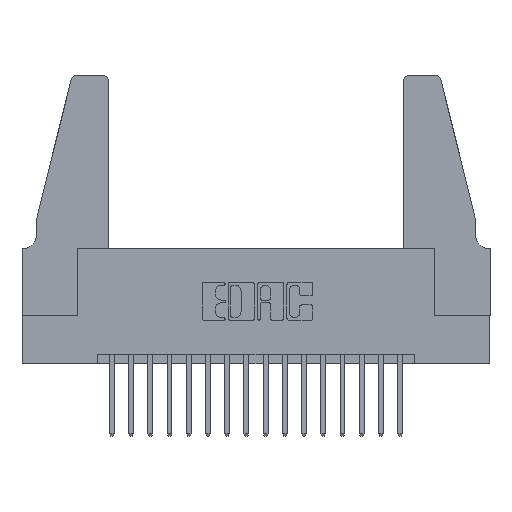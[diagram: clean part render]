
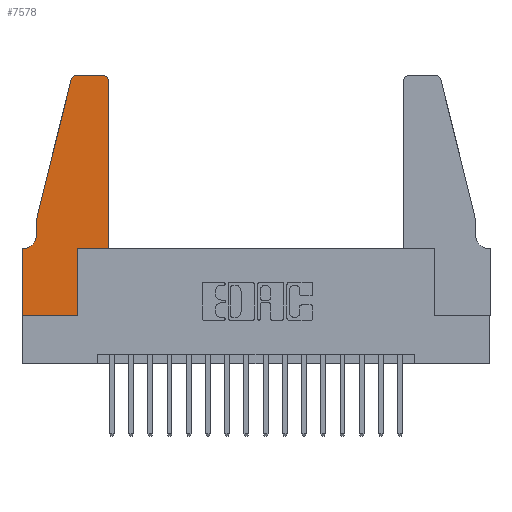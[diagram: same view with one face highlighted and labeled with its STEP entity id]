
A CAD part, top view. The second image highlights one B-rep face of the part: STEP entity #7578.
In plain terms, the highlighted planar face has unit normal (0, 0, 1).
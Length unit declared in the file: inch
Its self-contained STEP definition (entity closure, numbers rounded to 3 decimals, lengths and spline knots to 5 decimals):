
#6 = CARTESIAN_POINT ( 'NONE',  ( 0.0755, 0.5, 0.37 ) ) ;
#129 = CARTESIAN_POINT ( 'NONE',  ( 0.4205, 1.22, 0.37 ) ) ;
#446 = ORIENTED_EDGE ( 'NONE', *, *, #8183, .T. ) ;
#811 = CARTESIAN_POINT ( 'NONE',  ( 0., 0.35, 0.37 ) ) ;
#850 = CARTESIAN_POINT ( 'NONE',  ( 0.4205, 1.25, 0.37 ) ) ;
#881 = VECTOR ( 'NONE', #11920, 39.37008 ) ;
#1114 = CARTESIAN_POINT ( 'NONE',  ( 0.284, 1.22, 0.37 ) ) ;
#1154 = ORIENTED_EDGE ( 'NONE', *, *, #18149, .T. ) ;
#1182 = CARTESIAN_POINT ( 'NONE',  ( 0.4505, 0.35, 0.37 ) ) ;
#1520 = DIRECTION ( 'NONE',  ( 1., 0., 0. ) ) ;
#1636 = EDGE_CURVE ( 'NONE', #12787, #14306, #3996, .T. ) ;
#1684 = LINE ( 'NONE', #9466, #16262 ) ;
#1925 = EDGE_CURVE ( 'NONE', #4244, #3979, #17481, .T. ) ;
#2130 = CARTESIAN_POINT ( 'NONE',  ( 0., 0.35, 0.37 ) ) ;
#2363 = VECTOR ( 'NONE', #8413, 39.37008 ) ;
#2592 = CARTESIAN_POINT ( 'NONE',  ( 0.0055, 0.35, 0.37 ) ) ;
#2676 = CARTESIAN_POINT ( 'NONE',  ( 0.2865, 0.35, 0.37 ) ) ;
#2794 = CARTESIAN_POINT ( 'NONE',  ( 0.284, 1.25, 0.37 ) ) ;
#2969 = AXIS2_PLACEMENT_3D ( 'NONE', #1114, #8069, #10960 ) ;
#3422 = ORIENTED_EDGE ( 'NONE', *, *, #1636, .T. ) ;
#3979 = VERTEX_POINT ( 'NONE', #11394 ) ;
#3996 = LINE ( 'NONE', #12353, #13262 ) ;
#4066 = DIRECTION ( 'NONE',  ( 0., 1., 0. ) ) ;
#4141 = ORIENTED_EDGE ( 'NONE', *, *, #5455, .T. ) ;
#4175 = CARTESIAN_POINT ( 'NONE',  ( 0.25487, 1.22718, 0.37 ) ) ;
#4244 = VERTEX_POINT ( 'NONE', #1182 ) ;
#4346 = EDGE_CURVE ( 'NONE', #7268, #17238, #17404, .T. ) ;
#4402 = CARTESIAN_POINT ( 'NONE',  ( 0.0755, 0.42, 0.37 ) ) ;
#4586 = LINE ( 'NONE', #17491, #881 ) ;
#4915 = PLANE ( 'NONE',  #17980 ) ;
#5394 = VECTOR ( 'NONE', #4066, 39.37008 ) ;
#5455 = EDGE_CURVE ( 'NONE', #15726, #9981, #13923, .T. ) ;
#5701 = CARTESIAN_POINT ( 'NONE',  ( 0.0055, 0.42, 0.37 ) ) ;
#5777 = LINE ( 'NONE', #5840, #15089 ) ;
#5840 = CARTESIAN_POINT ( 'NONE',  ( 0.0755, 0.5, 0.37 ) ) ;
#5896 = CARTESIAN_POINT ( 'NONE',  ( 0., 0., 0.37 ) ) ;
#6059 = ORIENTED_EDGE ( 'NONE', *, *, #4346, .T. ) ;
#6671 = ORIENTED_EDGE ( 'NONE', *, *, #8958, .T. ) ;
#6711 = CARTESIAN_POINT ( 'NONE',  ( 0.4505, 0.35, 0.37 ) ) ;
#6892 = EDGE_CURVE ( 'NONE', #8736, #8867, #4586, .T. ) ;
#7268 = VERTEX_POINT ( 'NONE', #2592 ) ;
#7578 = ADVANCED_FACE ( 'NONE', ( #15820 ), #4915, .T. ) ;
#8048 = CARTESIAN_POINT ( 'NONE',  ( 0.2865, 0.35, 0.37 ) ) ;
#8069 = DIRECTION ( 'NONE',  ( 0., 0., 1. ) ) ;
#8148 = VECTOR ( 'NONE', #16765, 39.37008 ) ;
#8183 = EDGE_CURVE ( 'NONE', #8867, #10814, #10039, .T. ) ;
#8195 = EDGE_CURVE ( 'NONE', #17238, #12787, #1684, .T. ) ;
#8413 = DIRECTION ( 'NONE',  ( 1., 0., 0. ) ) ;
#8728 = VERTEX_POINT ( 'NONE', #8048 ) ;
#8736 = VERTEX_POINT ( 'NONE', #850 ) ;
#8867 = VERTEX_POINT ( 'NONE', #2794 ) ;
#8958 = EDGE_CURVE ( 'NONE', #14306, #8728, #9372, .T. ) ;
#9372 = LINE ( 'NONE', #2676, #5394 ) ;
#9466 = CARTESIAN_POINT ( 'NONE',  ( 0., 0., 0.37 ) ) ;
#9530 = DIRECTION ( 'NONE',  ( 0., -1., 0. ) ) ;
#9537 = EDGE_CURVE ( 'NONE', #9981, #7268, #10000, .T. ) ;
#9835 = LINE ( 'NONE', #12566, #2363 ) ;
#9981 = VERTEX_POINT ( 'NONE', #4402 ) ;
#10000 = CIRCLE ( 'NONE', #14908, 0.07 ) ;
#10039 = CIRCLE ( 'NONE', #2969, 0.03 ) ;
#10134 = ORIENTED_EDGE ( 'NONE', *, *, #1925, .T. ) ;
#10814 = VERTEX_POINT ( 'NONE', #4175 ) ;
#10960 = DIRECTION ( 'NONE',  ( 1., 0., 0. ) ) ;
#11394 = CARTESIAN_POINT ( 'NONE',  ( 0.4505, 1.22, 0.37 ) ) ;
#11684 = DIRECTION ( 'NONE',  ( -1., 0., 0. ) ) ;
#11920 = DIRECTION ( 'NONE',  ( -1., 0., 0. ) ) ;
#11992 = AXIS2_PLACEMENT_3D ( 'NONE', #129, #12857, #1520 ) ;
#12176 = VECTOR ( 'NONE', #12355, 39.37008 ) ;
#12353 = CARTESIAN_POINT ( 'NONE',  ( 0., 0., 0.37 ) ) ;
#12355 = DIRECTION ( 'NONE',  ( 0., 1., 0. ) ) ;
#12366 = EDGE_LOOP ( 'NONE', ( #12546, #446, #1154, #4141, #17890, #6059, #16382, #3422, #6671, #12944, #10134, #13856 ) ) ;
#12546 = ORIENTED_EDGE ( 'NONE', *, *, #6892, .T. ) ;
#12566 = CARTESIAN_POINT ( 'NONE',  ( 0.4505, 0.35, 0.37 ) ) ;
#12585 = CARTESIAN_POINT ( 'NONE',  ( 0.0755, 0.5, 0.37 ) ) ;
#12787 = VERTEX_POINT ( 'NONE', #5896 ) ;
#12857 = DIRECTION ( 'NONE',  ( 0., 0., 1. ) ) ;
#12944 = ORIENTED_EDGE ( 'NONE', *, *, #17320, .T. ) ;
#13155 = EDGE_CURVE ( 'NONE', #3979, #8736, #16408, .T. ) ;
#13262 = VECTOR ( 'NONE', #16579, 39.37008 ) ;
#13385 = CARTESIAN_POINT ( 'NONE',  ( 0.2865, 0., 0.37 ) ) ;
#13482 = DIRECTION ( 'NONE',  ( 1., 0., 0. ) ) ;
#13666 = CARTESIAN_POINT ( 'NONE',  ( 0.0755, 0.35, 0.37 ) ) ;
#13856 = ORIENTED_EDGE ( 'NONE', *, *, #13155, .T. ) ;
#13923 = LINE ( 'NONE', #6, #8148 ) ;
#14306 = VERTEX_POINT ( 'NONE', #13385 ) ;
#14908 = AXIS2_PLACEMENT_3D ( 'NONE', #5701, #15600, #11684 ) ;
#14922 = DIRECTION ( 'NONE',  ( 0., 0., 1. ) ) ;
#14960 = VECTOR ( 'NONE', #17962, 39.37008 ) ;
#15089 = VECTOR ( 'NONE', #17344, 39.37008 ) ;
#15600 = DIRECTION ( 'NONE',  ( 0., 0., -1. ) ) ;
#15726 = VERTEX_POINT ( 'NONE', #12585 ) ;
#15820 = FACE_OUTER_BOUND ( 'NONE', #12366, .T. ) ;
#16262 = VECTOR ( 'NONE', #9530, 39.37008 ) ;
#16382 = ORIENTED_EDGE ( 'NONE', *, *, #8195, .T. ) ;
#16408 = CIRCLE ( 'NONE', #11992, 0.03 ) ;
#16579 = DIRECTION ( 'NONE',  ( 1., 0., 0. ) ) ;
#16765 = DIRECTION ( 'NONE',  ( 0., -1., 0. ) ) ;
#17238 = VERTEX_POINT ( 'NONE', #2130 ) ;
#17320 = EDGE_CURVE ( 'NONE', #8728, #4244, #9835, .T. ) ;
#17344 = DIRECTION ( 'NONE',  ( -0.239, -0.971, 0. ) ) ;
#17404 = LINE ( 'NONE', #13666, #14960 ) ;
#17481 = LINE ( 'NONE', #6711, #12176 ) ;
#17491 = CARTESIAN_POINT ( 'NONE',  ( 0.2605, 1.25, 0.37 ) ) ;
#17890 = ORIENTED_EDGE ( 'NONE', *, *, #9537, .T. ) ;
#17962 = DIRECTION ( 'NONE',  ( -1., 0., 0. ) ) ;
#17980 = AXIS2_PLACEMENT_3D ( 'NONE', #811, #14922, #13482 ) ;
#18149 = EDGE_CURVE ( 'NONE', #10814, #15726, #5777, .T. ) ;
